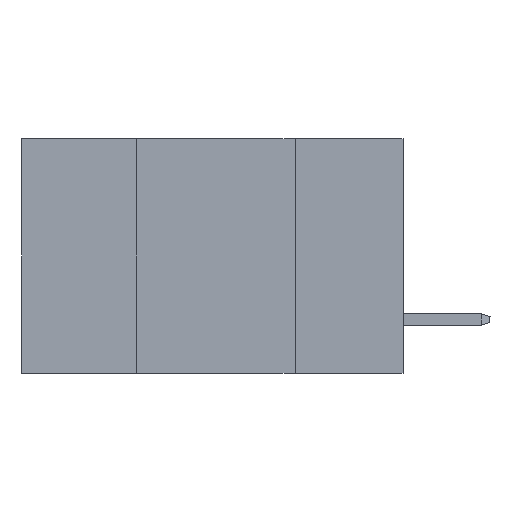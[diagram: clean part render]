
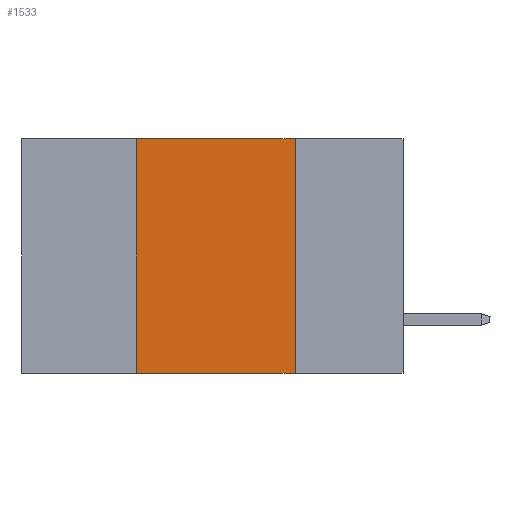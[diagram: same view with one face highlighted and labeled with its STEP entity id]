
A CAD part, left-side view. The second image highlights one B-rep face of the part: STEP entity #1533.
In plain terms, the highlighted planar face has unit normal (-1, 0, 0).
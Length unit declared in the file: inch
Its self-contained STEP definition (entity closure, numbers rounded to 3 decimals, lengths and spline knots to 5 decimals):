
#193 = CARTESIAN_POINT ( 'NONE',  ( 0., 0.6, 0. ) ) ;
#468 = EDGE_CURVE ( 'NONE', #2631, #4524, #9506, .T. ) ;
#548 = VECTOR ( 'NONE', #8550, 39.37008 ) ;
#661 = PLANE ( 'NONE',  #9147 ) ;
#1219 = ORIENTED_EDGE ( 'NONE', *, *, #10031, .F. ) ;
#1344 = DIRECTION ( 'NONE',  ( 0., 0., -1. ) ) ;
#1533 = ADVANCED_FACE ( 'NONE', ( #7421 ), #661, .F. ) ;
#2476 = ORIENTED_EDGE ( 'NONE', *, *, #468, .T. ) ;
#2631 = VERTEX_POINT ( 'NONE', #3252 ) ;
#3143 = DIRECTION ( 'NONE',  ( 0., -1., 0. ) ) ;
#3252 = CARTESIAN_POINT ( 'NONE',  ( 0., 0.42, -0.37 ) ) ;
#3597 = CARTESIAN_POINT ( 'NONE',  ( 0., 0.42, 0. ) ) ;
#3786 = DIRECTION ( 'NONE',  ( 0., 0., 1. ) ) ;
#4179 = VECTOR ( 'NONE', #3786, 39.37008 ) ;
#4524 = VERTEX_POINT ( 'NONE', #5542 ) ;
#4562 = DIRECTION ( 'NONE',  ( 1., 0., 0. ) ) ;
#4834 = ORIENTED_EDGE ( 'NONE', *, *, #9081, .F. ) ;
#5407 = VECTOR ( 'NONE', #1344, 39.37008 ) ;
#5542 = CARTESIAN_POINT ( 'NONE',  ( 0., 0.17, -0.37 ) ) ;
#5546 = CARTESIAN_POINT ( 'NONE',  ( 0., 0.6, -0.37 ) ) ;
#5957 = LINE ( 'NONE', #12004, #5407 ) ;
#6585 = CARTESIAN_POINT ( 'NONE',  ( 0., 0.6, 0. ) ) ;
#7250 = VECTOR ( 'NONE', #3143, 39.37008 ) ;
#7421 = FACE_OUTER_BOUND ( 'NONE', #11198, .T. ) ;
#8335 = VERTEX_POINT ( 'NONE', #11110 ) ;
#8550 = DIRECTION ( 'NONE',  ( 0., -1., 0. ) ) ;
#8741 = LINE ( 'NONE', #3597, #4179 ) ;
#8929 = LINE ( 'NONE', #193, #7250 ) ;
#9081 = EDGE_CURVE ( 'NONE', #2631, #8335, #8741, .T. ) ;
#9147 = AXIS2_PLACEMENT_3D ( 'NONE', #6585, #4562, #12470 ) ;
#9506 = LINE ( 'NONE', #5546, #548 ) ;
#10031 = EDGE_CURVE ( 'NONE', #12253, #4524, #5957, .T. ) ;
#10584 = EDGE_CURVE ( 'NONE', #8335, #12253, #8929, .T. ) ;
#11110 = CARTESIAN_POINT ( 'NONE',  ( 0., 0.42, 0. ) ) ;
#11198 = EDGE_LOOP ( 'NONE', ( #1219, #12383, #4834, #2476 ) ) ;
#11650 = CARTESIAN_POINT ( 'NONE',  ( 0., 0.17, 0. ) ) ;
#12004 = CARTESIAN_POINT ( 'NONE',  ( 0., 0.17, 0. ) ) ;
#12253 = VERTEX_POINT ( 'NONE', #11650 ) ;
#12383 = ORIENTED_EDGE ( 'NONE', *, *, #10584, .F. ) ;
#12470 = DIRECTION ( 'NONE',  ( 0., 0., -1. ) ) ;
